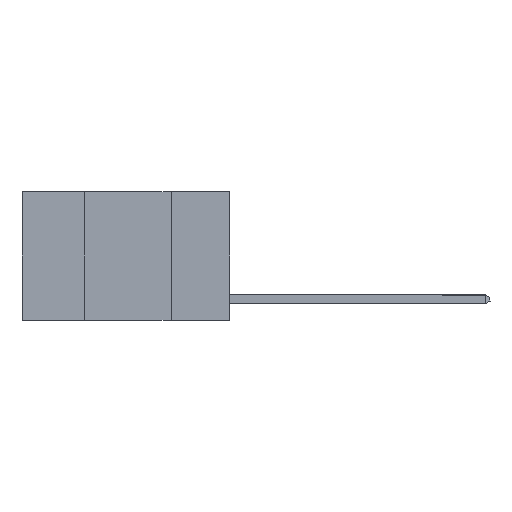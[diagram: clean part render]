
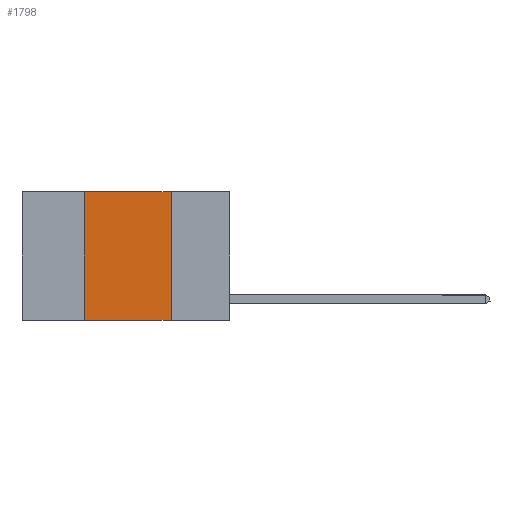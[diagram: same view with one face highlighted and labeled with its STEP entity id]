
A CAD part, left-side view. The second image highlights one B-rep face of the part: STEP entity #1798.
In plain terms, the highlighted planar face has unit normal (-1, 0, 0).
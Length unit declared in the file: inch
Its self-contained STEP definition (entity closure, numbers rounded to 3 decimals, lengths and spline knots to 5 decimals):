
#56 = CARTESIAN_POINT ( 'NONE',  ( 0., 0.6, 0. ) ) ;
#457 = CARTESIAN_POINT ( 'NONE',  ( 0., 0.42, -0.37 ) ) ;
#468 = VECTOR ( 'NONE', #4732, 39.37008 ) ;
#507 = DIRECTION ( 'NONE',  ( 0., 0., -1. ) ) ;
#930 = DIRECTION ( 'NONE',  ( 0., -1., 0. ) ) ;
#1798 = ADVANCED_FACE ( 'NONE', ( #7984 ), #4148, .F. ) ;
#2489 = DIRECTION ( 'NONE',  ( 0., 0., 1. ) ) ;
#3725 = VECTOR ( 'NONE', #507, 39.37008 ) ;
#4008 = LINE ( 'NONE', #56, #468 ) ;
#4042 = DIRECTION ( 'NONE',  ( 0., 0., -1. ) ) ;
#4103 = DIRECTION ( 'NONE',  ( 1., 0., 0. ) ) ;
#4148 = PLANE ( 'NONE',  #4505 ) ;
#4361 = CARTESIAN_POINT ( 'NONE',  ( 0., 0.6, 0. ) ) ;
#4400 = LINE ( 'NONE', #7025, #6020 ) ;
#4505 = AXIS2_PLACEMENT_3D ( 'NONE', #4361, #4103, #4042 ) ;
#4533 = ORIENTED_EDGE ( 'NONE', *, *, #7149, .F. ) ;
#4732 = DIRECTION ( 'NONE',  ( 0., -1., 0. ) ) ;
#4948 = LINE ( 'NONE', #7062, #8370 ) ;
#5091 = VERTEX_POINT ( 'NONE', #7364 ) ;
#5515 = LINE ( 'NONE', #7902, #3725 ) ;
#5572 = ORIENTED_EDGE ( 'NONE', *, *, #7459, .F. ) ;
#6020 = VECTOR ( 'NONE', #930, 39.37008 ) ;
#6242 = VERTEX_POINT ( 'NONE', #7102 ) ;
#6728 = EDGE_LOOP ( 'NONE', ( #4533, #5572, #8560, #7456 ) ) ;
#6989 = EDGE_CURVE ( 'NONE', #7091, #6242, #4948, .T. ) ;
#7025 = CARTESIAN_POINT ( 'NONE',  ( 0., 0.6, -0.37 ) ) ;
#7047 = CARTESIAN_POINT ( 'NONE',  ( 0., 0.17, 0. ) ) ;
#7062 = CARTESIAN_POINT ( 'NONE',  ( 0., 0.42, 0. ) ) ;
#7091 = VERTEX_POINT ( 'NONE', #457 ) ;
#7102 = CARTESIAN_POINT ( 'NONE',  ( 0., 0.42, 0. ) ) ;
#7149 = EDGE_CURVE ( 'NONE', #8570, #5091, #5515, .T. ) ;
#7364 = CARTESIAN_POINT ( 'NONE',  ( 0., 0.17, -0.37 ) ) ;
#7456 = ORIENTED_EDGE ( 'NONE', *, *, #8509, .T. ) ;
#7459 = EDGE_CURVE ( 'NONE', #6242, #8570, #4008, .T. ) ;
#7902 = CARTESIAN_POINT ( 'NONE',  ( 0., 0.17, 0. ) ) ;
#7984 = FACE_OUTER_BOUND ( 'NONE', #6728, .T. ) ;
#8370 = VECTOR ( 'NONE', #2489, 39.37008 ) ;
#8509 = EDGE_CURVE ( 'NONE', #7091, #5091, #4400, .T. ) ;
#8560 = ORIENTED_EDGE ( 'NONE', *, *, #6989, .F. ) ;
#8570 = VERTEX_POINT ( 'NONE', #7047 ) ;
